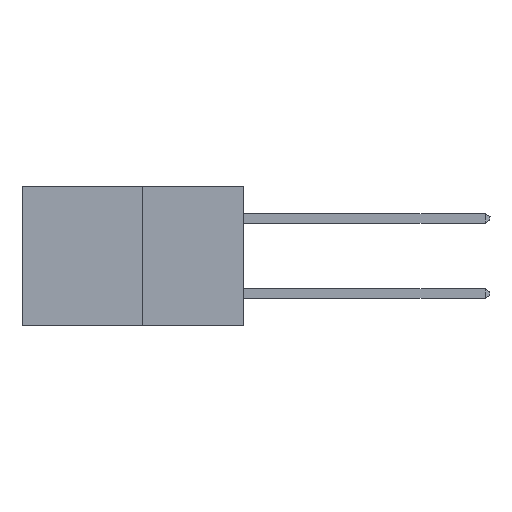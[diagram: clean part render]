
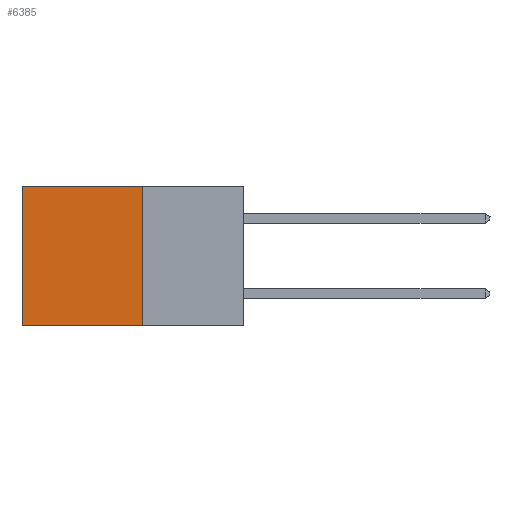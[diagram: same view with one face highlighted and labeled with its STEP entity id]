
A CAD part, left-side view. The second image highlights one B-rep face of the part: STEP entity #6385.
In plain terms, the highlighted planar face has unit normal (-1, 0, 0).
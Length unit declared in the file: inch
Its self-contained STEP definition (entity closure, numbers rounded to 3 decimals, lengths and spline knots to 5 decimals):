
#682 = AXIS2_PLACEMENT_3D ( 'NONE', #19022, #19130, #5191 ) ;
#3356 = FACE_OUTER_BOUND ( 'NONE', #24258, .T. ) ;
#3405 = DIRECTION ( 'NONE',  ( 0., 0., -1. ) ) ;
#4110 = ORIENTED_EDGE ( 'NONE', *, *, #26209, .T. ) ;
#4215 = ORIENTED_EDGE ( 'NONE', *, *, #24466, .F. ) ;
#5093 = VECTOR ( 'NONE', #3405, 39.37008 ) ;
#5191 = DIRECTION ( 'NONE',  ( 0., 0., -1. ) ) ;
#6385 = ADVANCED_FACE ( 'NONE', ( #3356 ), #16847, .F. ) ;
#6774 = ORIENTED_EDGE ( 'NONE', *, *, #8449, .F. ) ;
#7983 = VERTEX_POINT ( 'NONE', #17647 ) ;
#8200 = CARTESIAN_POINT ( 'NONE',  ( 0.277, 0.59, -0.37 ) ) ;
#8449 = EDGE_CURVE ( 'NONE', #17129, #7983, #13910, .T. ) ;
#8800 = DIRECTION ( 'NONE',  ( 0., 1., 0. ) ) ;
#12235 = LINE ( 'NONE', #20307, #18361 ) ;
#12293 = CARTESIAN_POINT ( 'NONE',  ( 0.277, 0.59, -0.37 ) ) ;
#13218 = VERTEX_POINT ( 'NONE', #18091 ) ;
#13333 = CARTESIAN_POINT ( 'NONE',  ( 0.277, 0.27, -0.37 ) ) ;
#13886 = CARTESIAN_POINT ( 'NONE',  ( 0.277, 0.27, 0. ) ) ;
#13910 = LINE ( 'NONE', #13333, #25425 ) ;
#14474 = LINE ( 'NONE', #13886, #25993 ) ;
#16196 = DIRECTION ( 'NONE',  ( 0., 1., 0. ) ) ;
#16847 = PLANE ( 'NONE',  #682 ) ;
#17129 = VERTEX_POINT ( 'NONE', #25718 ) ;
#17647 = CARTESIAN_POINT ( 'NONE',  ( 0.277, 0.27, -0.37 ) ) ;
#17951 = DIRECTION ( 'NONE',  ( 0., 0., -1. ) ) ;
#18091 = CARTESIAN_POINT ( 'NONE',  ( 0.277, 0.59, 0. ) ) ;
#18218 = LINE ( 'NONE', #8200, #5093 ) ;
#18361 = VECTOR ( 'NONE', #8800, 39.37008 ) ;
#18934 = EDGE_CURVE ( 'NONE', #17129, #13218, #14474, .T. ) ;
#19022 = CARTESIAN_POINT ( 'NONE',  ( 0.277, 0.27, -0.37 ) ) ;
#19130 = DIRECTION ( 'NONE',  ( 1., 0., 0. ) ) ;
#20307 = CARTESIAN_POINT ( 'NONE',  ( 0.277, 0.27, -0.37 ) ) ;
#24258 = EDGE_LOOP ( 'NONE', ( #4110, #4215, #6774, #26740 ) ) ;
#24466 = EDGE_CURVE ( 'NONE', #7983, #26056, #12235, .T. ) ;
#25425 = VECTOR ( 'NONE', #17951, 39.37008 ) ;
#25718 = CARTESIAN_POINT ( 'NONE',  ( 0.277, 0.27, 0. ) ) ;
#25993 = VECTOR ( 'NONE', #16196, 39.37008 ) ;
#26056 = VERTEX_POINT ( 'NONE', #12293 ) ;
#26209 = EDGE_CURVE ( 'NONE', #13218, #26056, #18218, .T. ) ;
#26740 = ORIENTED_EDGE ( 'NONE', *, *, #18934, .T. ) ;
